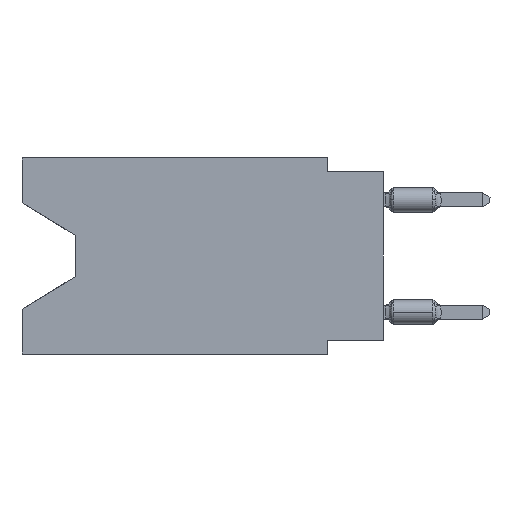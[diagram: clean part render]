
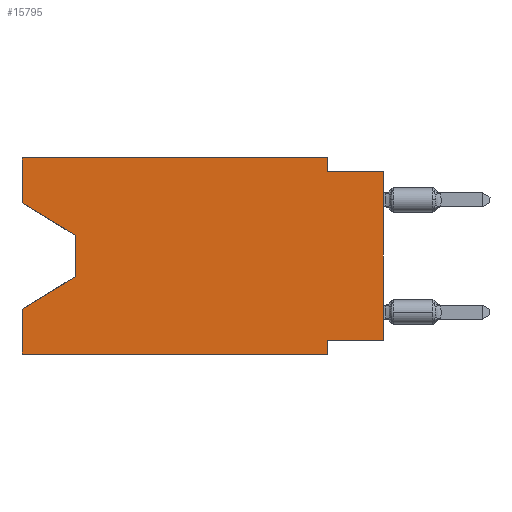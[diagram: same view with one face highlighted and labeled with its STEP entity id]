
A CAD part, left-side view. The second image highlights one B-rep face of the part: STEP entity #15795.
In plain terms, the highlighted planar face has unit normal (-1, 0, 0).
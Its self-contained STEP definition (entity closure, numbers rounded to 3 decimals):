
#99 = DIRECTION ( 'NONE',  ( 0., -1., 0. ) ) ;
#572 = CARTESIAN_POINT ( 'NONE',  ( 0., 16.383, 0. ) ) ;
#876 = EDGE_CURVE ( 'NONE', #11045, #6362, #15748, .T. ) ;
#1012 = CARTESIAN_POINT ( 'NONE',  ( 0., 16.383, -2.038 ) ) ;
#1221 = VECTOR ( 'NONE', #19404, 1000. ) ;
#1854 = LINE ( 'NONE', #572, #9842 ) ;
#2082 = CARTESIAN_POINT ( 'NONE',  ( 0., 16.383, -8.89 ) ) ;
#2084 = CARTESIAN_POINT ( 'NONE',  ( 0., 0., -0.635 ) ) ;
#2157 = ORIENTED_EDGE ( 'NONE', *, *, #15760, .T. ) ;
#2281 = CARTESIAN_POINT ( 'NONE',  ( 0., 0., -8.255 ) ) ;
#2306 = VECTOR ( 'NONE', #14125, 1000. ) ;
#2397 = DIRECTION ( 'NONE',  ( 0., 0., -1. ) ) ;
#2510 = CARTESIAN_POINT ( 'NONE',  ( 0., 16.383, 0. ) ) ;
#2571 = ORIENTED_EDGE ( 'NONE', *, *, #876, .T. ) ;
#2585 = VECTOR ( 'NONE', #8759, 1000. ) ;
#2781 = CARTESIAN_POINT ( 'NONE',  ( 0., 2.54, 0. ) ) ;
#3059 = CARTESIAN_POINT ( 'NONE',  ( 0., 13.97, -5.385 ) ) ;
#3133 = VERTEX_POINT ( 'NONE', #2781 ) ;
#3260 = VECTOR ( 'NONE', #9658, 1000. ) ;
#3529 = ORIENTED_EDGE ( 'NONE', *, *, #12884, .T. ) ;
#3941 = EDGE_CURVE ( 'NONE', #14888, #9593, #1854, .T. ) ;
#4371 = VERTEX_POINT ( 'NONE', #4456 ) ;
#4456 = CARTESIAN_POINT ( 'NONE',  ( 0., 2.54, -8.255 ) ) ;
#4876 = ORIENTED_EDGE ( 'NONE', *, *, #10056, .F. ) ;
#4961 = CARTESIAN_POINT ( 'NONE',  ( 0., 16.383, -6.852 ) ) ;
#5013 = EDGE_CURVE ( 'NONE', #4371, #19529, #20136, .T. ) ;
#5063 = VECTOR ( 'NONE', #17801, 1000. ) ;
#5092 = ORIENTED_EDGE ( 'NONE', *, *, #17627, .T. ) ;
#5247 = VECTOR ( 'NONE', #2397, 1000. ) ;
#5518 = CARTESIAN_POINT ( 'NONE',  ( 0., 16.383, 0. ) ) ;
#5935 = FACE_OUTER_BOUND ( 'NONE', #13429, .T. ) ;
#6224 = LINE ( 'NONE', #14832, #6642 ) ;
#6362 = VERTEX_POINT ( 'NONE', #13691 ) ;
#6491 = LINE ( 'NONE', #9711, #5063 ) ;
#6642 = VECTOR ( 'NONE', #99, 1000. ) ;
#6850 = ORIENTED_EDGE ( 'NONE', *, *, #16761, .F. ) ;
#7353 = DIRECTION ( 'NONE',  ( 0., -0.855, -0.519 ) ) ;
#7386 = EDGE_CURVE ( 'NONE', #11045, #17037, #13709, .T. ) ;
#7436 = VERTEX_POINT ( 'NONE', #10171 ) ;
#7553 = ORIENTED_EDGE ( 'NONE', *, *, #11979, .T. ) ;
#7654 = DIRECTION ( 'NONE',  ( 0., 0., -1. ) ) ;
#8734 = CARTESIAN_POINT ( 'NONE',  ( 0., 2.54, -8.89 ) ) ;
#8759 = DIRECTION ( 'NONE',  ( 0., 0., 1. ) ) ;
#8904 = CARTESIAN_POINT ( 'NONE',  ( 0., 2.54, 0. ) ) ;
#9063 = DIRECTION ( 'NONE',  ( 1., 0., 0. ) ) ;
#9074 = VECTOR ( 'NONE', #19402, 1000. ) ;
#9593 = VERTEX_POINT ( 'NONE', #4961 ) ;
#9658 = DIRECTION ( 'NONE',  ( 0., 0., 1. ) ) ;
#9711 = CARTESIAN_POINT ( 'NONE',  ( 0., 16.383, 0. ) ) ;
#9837 = ORIENTED_EDGE ( 'NONE', *, *, #5013, .F. ) ;
#9842 = VECTOR ( 'NONE', #19914, 1000. ) ;
#10056 = EDGE_CURVE ( 'NONE', #13758, #4371, #19994, .T. ) ;
#10171 = CARTESIAN_POINT ( 'NONE',  ( 0., 13.97, -5.385 ) ) ;
#10459 = VECTOR ( 'NONE', #15204, 1000. ) ;
#10479 = VERTEX_POINT ( 'NONE', #12416 ) ;
#10543 = AXIS2_PLACEMENT_3D ( 'NONE', #2510, #9063, #7654 ) ;
#10699 = VECTOR ( 'NONE', #7353, 1000. ) ;
#10892 = CARTESIAN_POINT ( 'NONE',  ( 0., 16.383, 0. ) ) ;
#11045 = VERTEX_POINT ( 'NONE', #19673 ) ;
#11528 = CARTESIAN_POINT ( 'NONE',  ( 0., 2.54, -8.89 ) ) ;
#11979 = EDGE_CURVE ( 'NONE', #7436, #9593, #20992, .T. ) ;
#12157 = EDGE_CURVE ( 'NONE', #10479, #19982, #20035, .T. ) ;
#12231 = ORIENTED_EDGE ( 'NONE', *, *, #7386, .F. ) ;
#12416 = CARTESIAN_POINT ( 'NONE',  ( 0., 2.54, -0.635 ) ) ;
#12610 = PLANE ( 'NONE',  #10543 ) ;
#12884 = EDGE_CURVE ( 'NONE', #13758, #19982, #13208, .T. ) ;
#13160 = EDGE_CURVE ( 'NONE', #3133, #10479, #20997, .T. ) ;
#13208 = LINE ( 'NONE', #16218, #3260 ) ;
#13429 = EDGE_LOOP ( 'NONE', ( #2571, #2157, #7553, #17494, #5092, #9837, #4876, #3529, #14850, #17847, #6850, #12231 ) ) ;
#13691 = CARTESIAN_POINT ( 'NONE',  ( 0., 13.97, -3.505 ) ) ;
#13709 = LINE ( 'NONE', #5518, #2585 ) ;
#13758 = VERTEX_POINT ( 'NONE', #2281 ) ;
#13920 = LINE ( 'NONE', #17133, #2306 ) ;
#14125 = DIRECTION ( 'NONE',  ( 0., 0., -1. ) ) ;
#14832 = CARTESIAN_POINT ( 'NONE',  ( 0., 16.383, -8.89 ) ) ;
#14850 = ORIENTED_EDGE ( 'NONE', *, *, #12157, .F. ) ;
#14888 = VERTEX_POINT ( 'NONE', #2082 ) ;
#15195 = VECTOR ( 'NONE', #16990, 1000. ) ;
#15204 = DIRECTION ( 'NONE',  ( 0., -1., 0. ) ) ;
#15748 = LINE ( 'NONE', #1012, #10699 ) ;
#15760 = EDGE_CURVE ( 'NONE', #6362, #7436, #13920, .T. ) ;
#15795 = ADVANCED_FACE ( 'NONE', ( #5935 ), #12610, .F. ) ;
#16218 = CARTESIAN_POINT ( 'NONE',  ( 0., 0., 0. ) ) ;
#16761 = EDGE_CURVE ( 'NONE', #17037, #3133, #6491, .T. ) ;
#16990 = DIRECTION ( 'NONE',  ( 0., 1., 0. ) ) ;
#17037 = VERTEX_POINT ( 'NONE', #10892 ) ;
#17133 = CARTESIAN_POINT ( 'NONE',  ( 0., 13.97, -3.505 ) ) ;
#17494 = ORIENTED_EDGE ( 'NONE', *, *, #3941, .F. ) ;
#17627 = EDGE_CURVE ( 'NONE', #14888, #19529, #6224, .T. ) ;
#17801 = DIRECTION ( 'NONE',  ( 0., -1., 0. ) ) ;
#17847 = ORIENTED_EDGE ( 'NONE', *, *, #13160, .F. ) ;
#18715 = CARTESIAN_POINT ( 'NONE',  ( 0., 0., -8.255 ) ) ;
#19402 = DIRECTION ( 'NONE',  ( 0., 0.855, -0.519 ) ) ;
#19404 = DIRECTION ( 'NONE',  ( 0., 0., -1. ) ) ;
#19529 = VERTEX_POINT ( 'NONE', #11528 ) ;
#19673 = CARTESIAN_POINT ( 'NONE',  ( 0., 16.383, -2.038 ) ) ;
#19676 = CARTESIAN_POINT ( 'NONE',  ( 0., 0., -0.635 ) ) ;
#19914 = DIRECTION ( 'NONE',  ( 0., 0., 1. ) ) ;
#19982 = VERTEX_POINT ( 'NONE', #19676 ) ;
#19994 = LINE ( 'NONE', #18715, #15195 ) ;
#20035 = LINE ( 'NONE', #2084, #10459 ) ;
#20136 = LINE ( 'NONE', #8734, #5247 ) ;
#20992 = LINE ( 'NONE', #3059, #9074 ) ;
#20997 = LINE ( 'NONE', #8904, #1221 ) ;
